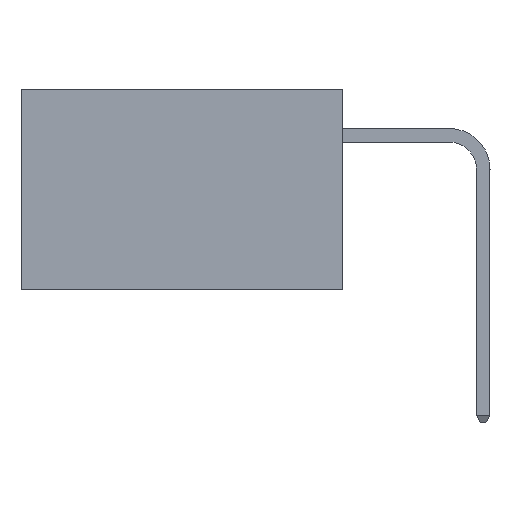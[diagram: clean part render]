
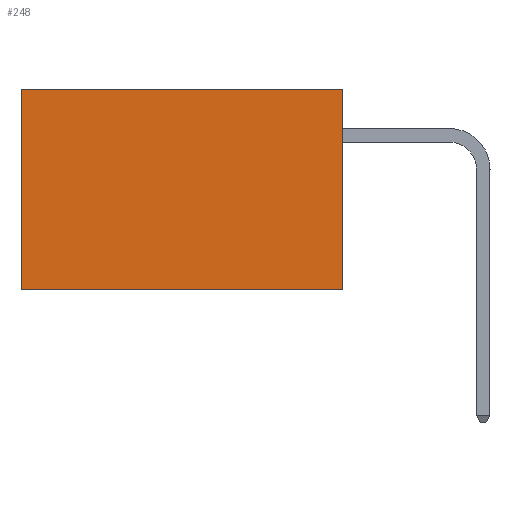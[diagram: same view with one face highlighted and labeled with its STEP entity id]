
A CAD part, left-side view. The second image highlights one B-rep face of the part: STEP entity #248.
In plain terms, the highlighted planar face has unit normal (-1, 0, 0).
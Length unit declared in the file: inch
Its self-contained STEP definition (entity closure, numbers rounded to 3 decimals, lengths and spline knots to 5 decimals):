
#248 = ADVANCED_FACE ( 'NONE', ( #18651 ), #25884, .F. ) ;
#1492 = VERTEX_POINT ( 'NONE', #1850 ) ;
#1850 = CARTESIAN_POINT ( 'NONE',  ( 0.277, 0., -0.37 ) ) ;
#3309 = DIRECTION ( 'NONE',  ( 1., 0., 0. ) ) ;
#3812 = VERTEX_POINT ( 'NONE', #9300 ) ;
#4399 = DIRECTION ( 'NONE',  ( 0., 0., -1. ) ) ;
#4424 = AXIS2_PLACEMENT_3D ( 'NONE', #21049, #3309, #4399 ) ;
#4602 = ORIENTED_EDGE ( 'NONE', *, *, #6414, .F. ) ;
#5476 = EDGE_CURVE ( 'NONE', #1492, #21972, #12430, .T. ) ;
#5954 = DIRECTION ( 'NONE',  ( 0., 1., 0. ) ) ;
#6414 = EDGE_CURVE ( 'NONE', #3812, #1492, #9745, .T. ) ;
#8549 = CARTESIAN_POINT ( 'NONE',  ( 0.277, 0.59, -0.37 ) ) ;
#8562 = LINE ( 'NONE', #8549, #19137 ) ;
#9084 = VECTOR ( 'NONE', #17473, 39.37008 ) ;
#9300 = CARTESIAN_POINT ( 'NONE',  ( 0.277, 0., 0. ) ) ;
#9745 = LINE ( 'NONE', #17203, #9084 ) ;
#10671 = DIRECTION ( 'NONE',  ( 0., 0., -1. ) ) ;
#12430 = LINE ( 'NONE', #24607, #18062 ) ;
#13226 = ORIENTED_EDGE ( 'NONE', *, *, #5476, .F. ) ;
#14208 = VERTEX_POINT ( 'NONE', #14304 ) ;
#14304 = CARTESIAN_POINT ( 'NONE',  ( 0.277, 0.59, 0. ) ) ;
#15578 = LINE ( 'NONE', #18609, #22558 ) ;
#17084 = EDGE_LOOP ( 'NONE', ( #17897, #13226, #4602, #17772 ) ) ;
#17203 = CARTESIAN_POINT ( 'NONE',  ( 0.277, 0., -0.37 ) ) ;
#17473 = DIRECTION ( 'NONE',  ( 0., 0., -1. ) ) ;
#17772 = ORIENTED_EDGE ( 'NONE', *, *, #21549, .T. ) ;
#17897 = ORIENTED_EDGE ( 'NONE', *, *, #24389, .T. ) ;
#18062 = VECTOR ( 'NONE', #23675, 39.37008 ) ;
#18609 = CARTESIAN_POINT ( 'NONE',  ( 0.277, 0., 0. ) ) ;
#18651 = FACE_OUTER_BOUND ( 'NONE', #17084, .T. ) ;
#19137 = VECTOR ( 'NONE', #10671, 39.37008 ) ;
#21049 = CARTESIAN_POINT ( 'NONE',  ( 0.277, 0., -0.37 ) ) ;
#21484 = CARTESIAN_POINT ( 'NONE',  ( 0.277, 0.59, -0.37 ) ) ;
#21549 = EDGE_CURVE ( 'NONE', #3812, #14208, #15578, .T. ) ;
#21972 = VERTEX_POINT ( 'NONE', #21484 ) ;
#22558 = VECTOR ( 'NONE', #5954, 39.37008 ) ;
#23675 = DIRECTION ( 'NONE',  ( 0., 1., 0. ) ) ;
#24389 = EDGE_CURVE ( 'NONE', #14208, #21972, #8562, .T. ) ;
#24607 = CARTESIAN_POINT ( 'NONE',  ( 0.277, 0., -0.37 ) ) ;
#25884 = PLANE ( 'NONE',  #4424 ) ;
